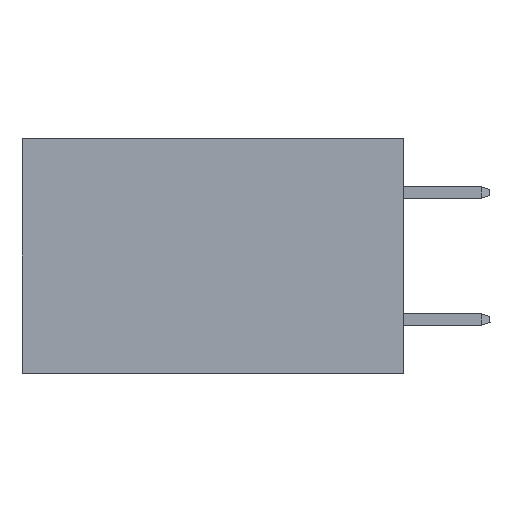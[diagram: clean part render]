
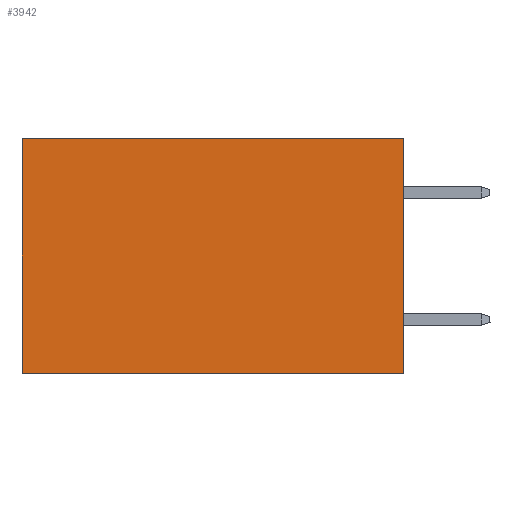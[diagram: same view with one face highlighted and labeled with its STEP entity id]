
A CAD part, left-side view. The second image highlights one B-rep face of the part: STEP entity #3942.
In plain terms, the highlighted planar face has unit normal (-1, 0, 0).
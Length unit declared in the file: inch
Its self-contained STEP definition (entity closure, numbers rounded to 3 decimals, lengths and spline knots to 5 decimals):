
#1047 = LINE ( 'NONE', #25999, #6592 ) ;
#2647 = AXIS2_PLACEMENT_3D ( 'NONE', #19893, #26167, #7481 ) ;
#3262 = PLANE ( 'NONE',  #2647 ) ;
#3871 = CARTESIAN_POINT ( 'NONE',  ( 0.2875, 0., 0. ) ) ;
#3942 = ADVANCED_FACE ( 'NONE', ( #21940 ), #3262, .F. ) ;
#3994 = VERTEX_POINT ( 'NONE', #4052 ) ;
#4004 = LINE ( 'NONE', #3871, #20296 ) ;
#4052 = CARTESIAN_POINT ( 'NONE',  ( 0.2875, 0., -0.37 ) ) ;
#4061 = CARTESIAN_POINT ( 'NONE',  ( 0.2875, 0.6, -0.37 ) ) ;
#4286 = EDGE_CURVE ( 'NONE', #14578, #7216, #1047, .T. ) ;
#6592 = VECTOR ( 'NONE', #11414, 39.37008 ) ;
#7216 = VERTEX_POINT ( 'NONE', #16439 ) ;
#7481 = DIRECTION ( 'NONE',  ( 0., 0., -1. ) ) ;
#8582 = ORIENTED_EDGE ( 'NONE', *, *, #12175, .F. ) ;
#10340 = LINE ( 'NONE', #18645, #15897 ) ;
#11414 = DIRECTION ( 'NONE',  ( 0., 1., 0. ) ) ;
#12175 = EDGE_CURVE ( 'NONE', #14578, #3994, #4004, .T. ) ;
#13241 = ORIENTED_EDGE ( 'NONE', *, *, #15558, .F. ) ;
#14030 = DIRECTION ( 'NONE',  ( 0., 0., -1. ) ) ;
#14336 = EDGE_LOOP ( 'NONE', ( #18647, #13241, #8582, #22603 ) ) ;
#14578 = VERTEX_POINT ( 'NONE', #23432 ) ;
#15558 = EDGE_CURVE ( 'NONE', #3994, #21440, #24689, .T. ) ;
#15897 = VECTOR ( 'NONE', #14030, 39.37008 ) ;
#16439 = CARTESIAN_POINT ( 'NONE',  ( 0.2875, 0.6, 0. ) ) ;
#18645 = CARTESIAN_POINT ( 'NONE',  ( 0.2875, 0.6, 0. ) ) ;
#18647 = ORIENTED_EDGE ( 'NONE', *, *, #21354, .T. ) ;
#19118 = VECTOR ( 'NONE', #26463, 39.37008 ) ;
#19893 = CARTESIAN_POINT ( 'NONE',  ( 0.2875, 0., 0. ) ) ;
#20296 = VECTOR ( 'NONE', #20630, 39.37008 ) ;
#20630 = DIRECTION ( 'NONE',  ( 0., 0., -1. ) ) ;
#21354 = EDGE_CURVE ( 'NONE', #7216, #21440, #10340, .T. ) ;
#21440 = VERTEX_POINT ( 'NONE', #4061 ) ;
#21940 = FACE_OUTER_BOUND ( 'NONE', #14336, .T. ) ;
#22242 = CARTESIAN_POINT ( 'NONE',  ( 0.2875, 0., -0.37 ) ) ;
#22603 = ORIENTED_EDGE ( 'NONE', *, *, #4286, .T. ) ;
#23432 = CARTESIAN_POINT ( 'NONE',  ( 0.2875, 0., 0. ) ) ;
#24689 = LINE ( 'NONE', #22242, #19118 ) ;
#25999 = CARTESIAN_POINT ( 'NONE',  ( 0.2875, 0., 0. ) ) ;
#26167 = DIRECTION ( 'NONE',  ( 1., 0., 0. ) ) ;
#26463 = DIRECTION ( 'NONE',  ( 0., 1., 0. ) ) ;
